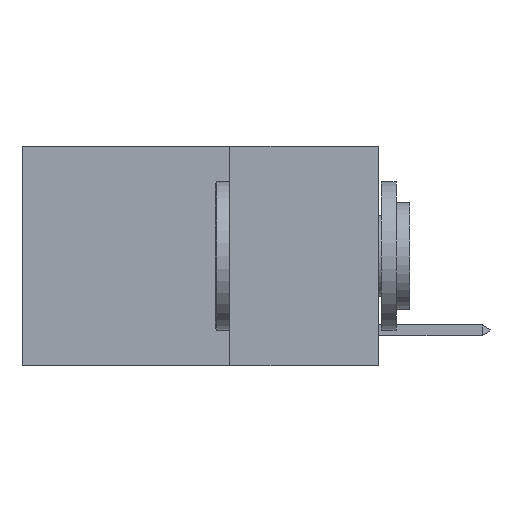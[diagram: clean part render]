
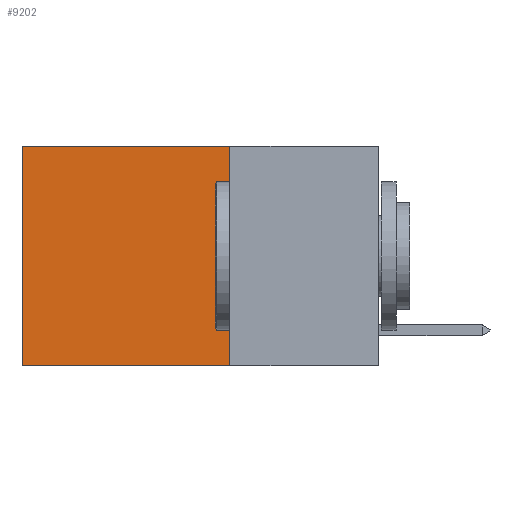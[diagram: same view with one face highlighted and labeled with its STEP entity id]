
A CAD part, left-side view. The second image highlights one B-rep face of the part: STEP entity #9202.
In plain terms, the highlighted planar face has unit normal (-1, 0, 0).
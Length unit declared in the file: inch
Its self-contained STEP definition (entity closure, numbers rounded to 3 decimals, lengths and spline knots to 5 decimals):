
#47 = DIRECTION ( 'NONE',  ( 1., 0., 0. ) ) ;
#141 = DIRECTION ( 'NONE',  ( 0., 1., 0. ) ) ;
#386 = EDGE_CURVE ( 'NONE', #7060, #14165, #7422, .T. ) ;
#492 = AXIS2_PLACEMENT_3D ( 'NONE', #12623, #47, #8089 ) ;
#681 = ORIENTED_EDGE ( 'NONE', *, *, #386, .F. ) ;
#1630 = LINE ( 'NONE', #11195, #4260 ) ;
#2020 = ORIENTED_EDGE ( 'NONE', *, *, #13785, .T. ) ;
#3818 = VECTOR ( 'NONE', #8535, 39.37008 ) ;
#3896 = LINE ( 'NONE', #9346, #12746 ) ;
#4260 = VECTOR ( 'NONE', #8968, 39.37008 ) ;
#5611 = DIRECTION ( 'NONE',  ( 0., 0., -1. ) ) ;
#6911 = PLANE ( 'NONE',  #492 ) ;
#6932 = LINE ( 'NONE', #14148, #3818 ) ;
#7060 = VERTEX_POINT ( 'NONE', #8366 ) ;
#7422 = LINE ( 'NONE', #12053, #10451 ) ;
#7489 = VERTEX_POINT ( 'NONE', #10305 ) ;
#7605 = VERTEX_POINT ( 'NONE', #9412 ) ;
#7903 = FACE_OUTER_BOUND ( 'NONE', #9897, .T. ) ;
#8089 = DIRECTION ( 'NONE',  ( 0., 0., -1. ) ) ;
#8245 = EDGE_CURVE ( 'NONE', #14165, #7605, #3896, .T. ) ;
#8366 = CARTESIAN_POINT ( 'NONE',  ( 0.2625, 0.25, 0. ) ) ;
#8535 = DIRECTION ( 'NONE',  ( 0., 1., 0. ) ) ;
#8968 = DIRECTION ( 'NONE',  ( 0., 0., -1. ) ) ;
#9202 = ADVANCED_FACE ( 'NONE', ( #7903 ), #6911, .F. ) ;
#9273 = ORIENTED_EDGE ( 'NONE', *, *, #11237, .T. ) ;
#9346 = CARTESIAN_POINT ( 'NONE',  ( 0.2625, 0.25, -0.37 ) ) ;
#9412 = CARTESIAN_POINT ( 'NONE',  ( 0.2625, 0.6, -0.37 ) ) ;
#9897 = EDGE_LOOP ( 'NONE', ( #2020, #12871, #681, #9273 ) ) ;
#10305 = CARTESIAN_POINT ( 'NONE',  ( 0.2625, 0.6, 0. ) ) ;
#10451 = VECTOR ( 'NONE', #5611, 39.37008 ) ;
#11195 = CARTESIAN_POINT ( 'NONE',  ( 0.2625, 0.6, 0. ) ) ;
#11237 = EDGE_CURVE ( 'NONE', #7060, #7489, #6932, .T. ) ;
#11894 = CARTESIAN_POINT ( 'NONE',  ( 0.2625, 0.25, -0.37 ) ) ;
#12053 = CARTESIAN_POINT ( 'NONE',  ( 0.2625, 0.25, 0. ) ) ;
#12623 = CARTESIAN_POINT ( 'NONE',  ( 0.2625, 0.25, 0. ) ) ;
#12746 = VECTOR ( 'NONE', #141, 39.37008 ) ;
#12871 = ORIENTED_EDGE ( 'NONE', *, *, #8245, .F. ) ;
#13785 = EDGE_CURVE ( 'NONE', #7489, #7605, #1630, .T. ) ;
#14148 = CARTESIAN_POINT ( 'NONE',  ( 0.2625, 0.25, 0. ) ) ;
#14165 = VERTEX_POINT ( 'NONE', #11894 ) ;
